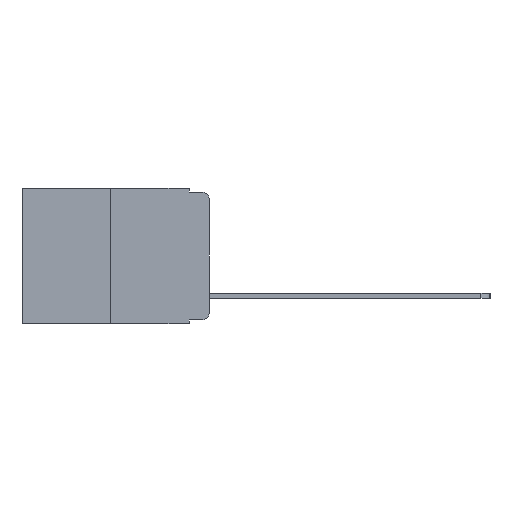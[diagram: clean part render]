
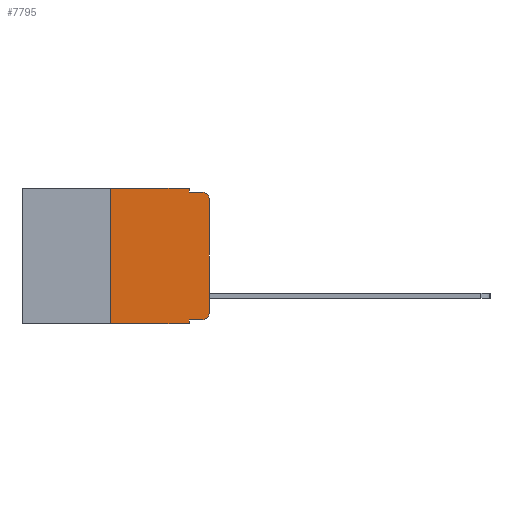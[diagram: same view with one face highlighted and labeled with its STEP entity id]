
A CAD part, left-side view. The second image highlights one B-rep face of the part: STEP entity #7795.
In plain terms, the highlighted planar face has unit normal (-1, 0, 0).
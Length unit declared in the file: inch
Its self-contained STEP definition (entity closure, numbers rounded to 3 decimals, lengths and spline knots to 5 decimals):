
#192 = VERTEX_POINT ( 'NONE', #926 ) ;
#241 = EDGE_CURVE ( 'NONE', #7001, #3936, #1003, .T. ) ;
#427 = LINE ( 'NONE', #10390, #11952 ) ;
#509 = DIRECTION ( 'NONE',  ( 0., -1., 0. ) ) ;
#591 = LINE ( 'NONE', #10562, #5925 ) ;
#693 = EDGE_CURVE ( 'NONE', #7001, #192, #7040, .T. ) ;
#759 = CARTESIAN_POINT ( 'NONE',  ( 0., 0.02, -0.01 ) ) ;
#824 = CARTESIAN_POINT ( 'NONE',  ( 0., 0.02, -0.333 ) ) ;
#832 = CARTESIAN_POINT ( 'NONE',  ( 0., 0.051, 0. ) ) ;
#857 = ORIENTED_EDGE ( 'NONE', *, *, #15594, .T. ) ;
#926 = CARTESIAN_POINT ( 'NONE',  ( 0., 0.051, -0.343 ) ) ;
#1003 = LINE ( 'NONE', #2158, #11872 ) ;
#1698 = CARTESIAN_POINT ( 'NONE',  ( 0., 0.051, -0.333 ) ) ;
#1880 = DIRECTION ( 'NONE',  ( 0., 0., -1. ) ) ;
#1939 = DIRECTION ( 'NONE',  ( 0., 0., 1. ) ) ;
#2029 = DIRECTION ( 'NONE',  ( 0., -1., 0. ) ) ;
#2102 = VECTOR ( 'NONE', #14869, 39.37008 ) ;
#2158 = CARTESIAN_POINT ( 'NONE',  ( 0., 0.051, -0.333 ) ) ;
#2201 = CARTESIAN_POINT ( 'NONE',  ( 0., 0., -0.313 ) ) ;
#2397 = VECTOR ( 'NONE', #2029, 39.37008 ) ;
#2610 = CARTESIAN_POINT ( 'NONE',  ( 0., 0.25, 0. ) ) ;
#2868 = VERTEX_POINT ( 'NONE', #4645 ) ;
#2871 = FACE_OUTER_BOUND ( 'NONE', #11249, .T. ) ;
#3589 = LINE ( 'NONE', #2610, #2102 ) ;
#3728 = VECTOR ( 'NONE', #1939, 39.37008 ) ;
#3844 = ORIENTED_EDGE ( 'NONE', *, *, #12476, .F. ) ;
#3936 = VERTEX_POINT ( 'NONE', #824 ) ;
#4258 = LINE ( 'NONE', #9253, #13348 ) ;
#4602 = ORIENTED_EDGE ( 'NONE', *, *, #7897, .F. ) ;
#4645 = CARTESIAN_POINT ( 'NONE',  ( 0., 0.25, -0.343 ) ) ;
#4939 = ORIENTED_EDGE ( 'NONE', *, *, #8374, .T. ) ;
#5475 = CARTESIAN_POINT ( 'NONE',  ( 0., 0.25, 0. ) ) ;
#5736 = DIRECTION ( 'NONE',  ( 0., 0., -1. ) ) ;
#5807 = DIRECTION ( 'NONE',  ( 0., 0., -1. ) ) ;
#5825 = DIRECTION ( 'NONE',  ( 0., -1., 0. ) ) ;
#5925 = VECTOR ( 'NONE', #6136, 39.37008 ) ;
#6041 = CIRCLE ( 'NONE', #9698, 0.02 ) ;
#6136 = DIRECTION ( 'NONE',  ( 0., 0., -1. ) ) ;
#6195 = EDGE_CURVE ( 'NONE', #10902, #8495, #427, .T. ) ;
#6276 = CARTESIAN_POINT ( 'NONE',  ( 0., 0., -0.03 ) ) ;
#6293 = ORIENTED_EDGE ( 'NONE', *, *, #6810, .F. ) ;
#6629 = DIRECTION ( 'NONE',  ( 1., 0., 0. ) ) ;
#6810 = EDGE_CURVE ( 'NONE', #2868, #10902, #3589, .T. ) ;
#7001 = VERTEX_POINT ( 'NONE', #1698 ) ;
#7040 = LINE ( 'NONE', #832, #15508 ) ;
#7298 = CIRCLE ( 'NONE', #14607, 0.02 ) ;
#7785 = DIRECTION ( 'NONE',  ( 0., 0., -1. ) ) ;
#7795 = ADVANCED_FACE ( 'NONE', ( #2871 ), #7857, .F. ) ;
#7857 = PLANE ( 'NONE',  #9953 ) ;
#7897 = EDGE_CURVE ( 'NONE', #9534, #15131, #13474, .T. ) ;
#8374 = EDGE_CURVE ( 'NONE', #11026, #15704, #15677, .T. ) ;
#8495 = VERTEX_POINT ( 'NONE', #15087 ) ;
#9013 = DIRECTION ( 'NONE',  ( -1., 0., 0. ) ) ;
#9253 = CARTESIAN_POINT ( 'NONE',  ( 0., 0.473, -0.343 ) ) ;
#9534 = VERTEX_POINT ( 'NONE', #9898 ) ;
#9695 = CARTESIAN_POINT ( 'NONE',  ( 0., 0., 0. ) ) ;
#9698 = AXIS2_PLACEMENT_3D ( 'NONE', #15232, #9013, #7785 ) ;
#9898 = CARTESIAN_POINT ( 'NONE',  ( 0., 0.051, -0.01 ) ) ;
#9953 = AXIS2_PLACEMENT_3D ( 'NONE', #12835, #6629, #1880 ) ;
#10068 = ORIENTED_EDGE ( 'NONE', *, *, #241, .T. ) ;
#10390 = CARTESIAN_POINT ( 'NONE',  ( 0., 0.473, 0. ) ) ;
#10562 = CARTESIAN_POINT ( 'NONE',  ( 0., 0.051, 0. ) ) ;
#10902 = VERTEX_POINT ( 'NONE', #5475 ) ;
#11026 = VERTEX_POINT ( 'NONE', #2201 ) ;
#11249 = EDGE_LOOP ( 'NONE', ( #4939, #15041, #4602, #3844, #15056, #6293, #857, #16150, #10068, #15945 ) ) ;
#11872 = VECTOR ( 'NONE', #5825, 39.37008 ) ;
#11952 = VECTOR ( 'NONE', #509, 39.37008 ) ;
#12476 = EDGE_CURVE ( 'NONE', #8495, #9534, #591, .T. ) ;
#12835 = CARTESIAN_POINT ( 'NONE',  ( 0., 0.473, 0. ) ) ;
#13348 = VECTOR ( 'NONE', #14244, 39.37008 ) ;
#13395 = CARTESIAN_POINT ( 'NONE',  ( 0., 0.051, -0.01 ) ) ;
#13474 = LINE ( 'NONE', #13395, #2397 ) ;
#14244 = DIRECTION ( 'NONE',  ( 0., -1., 0. ) ) ;
#14335 = DIRECTION ( 'NONE',  ( -1., 0., 0. ) ) ;
#14607 = AXIS2_PLACEMENT_3D ( 'NONE', #15649, #14335, #5736 ) ;
#14869 = DIRECTION ( 'NONE',  ( 0., 0., 1. ) ) ;
#15041 = ORIENTED_EDGE ( 'NONE', *, *, #15137, .T. ) ;
#15056 = ORIENTED_EDGE ( 'NONE', *, *, #6195, .F. ) ;
#15087 = CARTESIAN_POINT ( 'NONE',  ( 0., 0.051, 0. ) ) ;
#15131 = VERTEX_POINT ( 'NONE', #759 ) ;
#15137 = EDGE_CURVE ( 'NONE', #15704, #15131, #7298, .T. ) ;
#15232 = CARTESIAN_POINT ( 'NONE',  ( 0., 0.02, -0.313 ) ) ;
#15485 = EDGE_CURVE ( 'NONE', #3936, #11026, #6041, .T. ) ;
#15508 = VECTOR ( 'NONE', #5807, 39.37008 ) ;
#15594 = EDGE_CURVE ( 'NONE', #2868, #192, #4258, .T. ) ;
#15649 = CARTESIAN_POINT ( 'NONE',  ( 0., 0.02, -0.03 ) ) ;
#15677 = LINE ( 'NONE', #9695, #3728 ) ;
#15704 = VERTEX_POINT ( 'NONE', #6276 ) ;
#15945 = ORIENTED_EDGE ( 'NONE', *, *, #15485, .T. ) ;
#16150 = ORIENTED_EDGE ( 'NONE', *, *, #693, .F. ) ;
